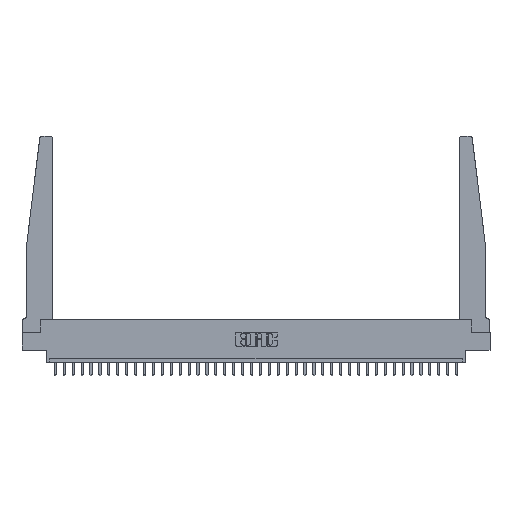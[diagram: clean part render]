
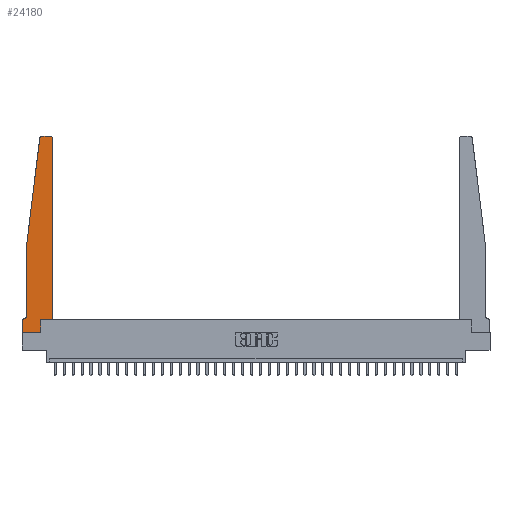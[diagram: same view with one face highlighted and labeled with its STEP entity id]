
A CAD part, top view. The second image highlights one B-rep face of the part: STEP entity #24180.
In plain terms, the highlighted planar face has unit normal (0, 0, 1).
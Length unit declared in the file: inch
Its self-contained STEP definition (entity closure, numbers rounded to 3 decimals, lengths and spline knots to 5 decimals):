
#249 = VERTEX_POINT ( 'NONE', #25269 ) ;
#447 = ORIENTED_EDGE ( 'NONE', *, *, #11841, .T. ) ;
#845 = CARTESIAN_POINT ( 'NONE',  ( 0.2605, 0.18, 0.37 ) ) ;
#974 = CARTESIAN_POINT ( 'NONE',  ( 0.27653, 2.75, 0.37 ) ) ;
#1027 = ORIENTED_EDGE ( 'NONE', *, *, #14362, .T. ) ;
#1041 = ORIENTED_EDGE ( 'NONE', *, *, #11023, .T. ) ;
#1573 = LINE ( 'NONE', #22048, #18857 ) ;
#1698 = CARTESIAN_POINT ( 'NONE',  ( 0.015, 0.1875, 0.37 ) ) ;
#2093 = ORIENTED_EDGE ( 'NONE', *, *, #29009, .T. ) ;
#2115 = VERTEX_POINT ( 'NONE', #1698 ) ;
#2901 = EDGE_CURVE ( 'NONE', #2115, #19477, #16508, .T. ) ;
#3150 = EDGE_CURVE ( 'NONE', #9063, #27293, #18668, .T. ) ;
#3406 = VECTOR ( 'NONE', #26445, 39.37008 ) ;
#3407 = ORIENTED_EDGE ( 'NONE', *, *, #17997, .T. ) ;
#3594 = LINE ( 'NONE', #24094, #30791 ) ;
#4368 = CARTESIAN_POINT ( 'NONE',  ( 0., 0., 0.37 ) ) ;
#4501 = DIRECTION ( 'NONE',  ( 1., 0., 0. ) ) ;
#6658 = LINE ( 'NONE', #21712, #22932 ) ;
#7038 = CARTESIAN_POINT ( 'NONE',  ( 0., 0.1875, 0.37 ) ) ;
#7677 = CARTESIAN_POINT ( 'NONE',  ( 0.2605, 0., 0.37 ) ) ;
#7689 = DIRECTION ( 'NONE',  ( 1., 0., 0. ) ) ;
#8015 = DIRECTION ( 'NONE',  ( 0., 0., 1. ) ) ;
#8926 = DIRECTION ( 'NONE',  ( -1., 0., 0. ) ) ;
#9063 = VERTEX_POINT ( 'NONE', #10203 ) ;
#9131 = AXIS2_PLACEMENT_3D ( 'NONE', #18800, #19141, #29138 ) ;
#9810 = VECTOR ( 'NONE', #16277, 39.37008 ) ;
#10203 = CARTESIAN_POINT ( 'NONE',  ( 0.425, 2.72, 0.37 ) ) ;
#10653 = LINE ( 'NONE', #18788, #18963 ) ;
#11023 = EDGE_CURVE ( 'NONE', #27715, #249, #14028, .T. ) ;
#11247 = CARTESIAN_POINT ( 'NONE',  ( 0.425, 0.18, 0.37 ) ) ;
#11837 = CARTESIAN_POINT ( 'NONE',  ( 0.425, 0.18, 0.37 ) ) ;
#11841 = EDGE_CURVE ( 'NONE', #27293, #32899, #18833, .T. ) ;
#12548 = AXIS2_PLACEMENT_3D ( 'NONE', #32112, #26361, #8926 ) ;
#14028 = LINE ( 'NONE', #11837, #29240 ) ;
#14362 = EDGE_CURVE ( 'NONE', #21719, #2115, #32006, .T. ) ;
#14790 = EDGE_CURVE ( 'NONE', #249, #9063, #18699, .T. ) ;
#14977 = PLANE ( 'NONE',  #32138 ) ;
#15306 = EDGE_CURVE ( 'NONE', #23309, #19709, #28999, .T. ) ;
#16064 = DIRECTION ( 'NONE',  ( 1., 0., 0. ) ) ;
#16275 = CARTESIAN_POINT ( 'NONE',  ( 0.395, 2.75, 0.37 ) ) ;
#16277 = DIRECTION ( 'NONE',  ( -1., 0., 0. ) ) ;
#16382 = VERTEX_POINT ( 'NONE', #7677 ) ;
#16490 = DIRECTION ( 'NONE',  ( 0., 1., 0. ) ) ;
#16508 = LINE ( 'NONE', #27013, #17019 ) ;
#16528 = EDGE_CURVE ( 'NONE', #19477, #22649, #3594, .T. ) ;
#17019 = VECTOR ( 'NONE', #32258, 39.37008 ) ;
#17597 = ORIENTED_EDGE ( 'NONE', *, *, #2901, .T. ) ;
#17843 = ORIENTED_EDGE ( 'NONE', *, *, #16528, .T. ) ;
#17997 = EDGE_CURVE ( 'NONE', #22649, #16382, #10653, .T. ) ;
#18668 = CIRCLE ( 'NONE', #26778, 0.03 ) ;
#18699 = LINE ( 'NONE', #11247, #27184 ) ;
#18788 = CARTESIAN_POINT ( 'NONE',  ( 0., 0., 0.37 ) ) ;
#18800 = CARTESIAN_POINT ( 'NONE',  ( 0.27653, 2.72, 0.37 ) ) ;
#18833 = LINE ( 'NONE', #21528, #9810 ) ;
#18857 = VECTOR ( 'NONE', #19178, 39.37008 ) ;
#18963 = VECTOR ( 'NONE', #16064, 39.37008 ) ;
#19141 = DIRECTION ( 'NONE',  ( 0., 0., 1. ) ) ;
#19178 = DIRECTION ( 'NONE',  ( 0., 1., 0. ) ) ;
#19477 = VERTEX_POINT ( 'NONE', #27939 ) ;
#19709 = VERTEX_POINT ( 'NONE', #28593 ) ;
#19768 = EDGE_LOOP ( 'NONE', ( #447, #24705, #22943, #21004, #1027, #17597, #17843, #3407, #2093, #1041, #32133, #27331 ) ) ;
#21004 = ORIENTED_EDGE ( 'NONE', *, *, #21642, .T. ) ;
#21528 = CARTESIAN_POINT ( 'NONE',  ( 0.25, 2.75, 0.37 ) ) ;
#21642 = EDGE_CURVE ( 'NONE', #19709, #21719, #6658, .T. ) ;
#21712 = CARTESIAN_POINT ( 'NONE',  ( 0.065, 1.25, 0.37 ) ) ;
#21719 = VERTEX_POINT ( 'NONE', #24272 ) ;
#22048 = CARTESIAN_POINT ( 'NONE',  ( 0.2605, 0.18, 0.37 ) ) ;
#22649 = VERTEX_POINT ( 'NONE', #4368 ) ;
#22777 = DIRECTION ( 'NONE',  ( 0., 0., 1. ) ) ;
#22932 = VECTOR ( 'NONE', #26808, 39.37008 ) ;
#22943 = ORIENTED_EDGE ( 'NONE', *, *, #15306, .T. ) ;
#23309 = VERTEX_POINT ( 'NONE', #30153 ) ;
#23715 = CIRCLE ( 'NONE', #9131, 0.03 ) ;
#24094 = CARTESIAN_POINT ( 'NONE',  ( 0., 0., 0.37 ) ) ;
#24180 = ADVANCED_FACE ( 'NONE', ( #27874 ), #14977, .T. ) ;
#24272 = CARTESIAN_POINT ( 'NONE',  ( 0.065, 0.2375, 0.37 ) ) ;
#24705 = ORIENTED_EDGE ( 'NONE', *, *, #29475, .T. ) ;
#25269 = CARTESIAN_POINT ( 'NONE',  ( 0.425, 0.18, 0.37 ) ) ;
#26361 = DIRECTION ( 'NONE',  ( 0., 0., -1. ) ) ;
#26445 = DIRECTION ( 'NONE',  ( -0.122, -0.992, 0. ) ) ;
#26615 = CARTESIAN_POINT ( 'NONE',  ( 0.065, 1.25, 0.37 ) ) ;
#26778 = AXIS2_PLACEMENT_3D ( 'NONE', #28679, #8015, #7689 ) ;
#26797 = DIRECTION ( 'NONE',  ( 0., -1., 0. ) ) ;
#26808 = DIRECTION ( 'NONE',  ( 0., -1., 0. ) ) ;
#27013 = CARTESIAN_POINT ( 'NONE',  ( 0.065, 0.1875, 0.37 ) ) ;
#27184 = VECTOR ( 'NONE', #16490, 39.37008 ) ;
#27293 = VERTEX_POINT ( 'NONE', #16275 ) ;
#27331 = ORIENTED_EDGE ( 'NONE', *, *, #3150, .T. ) ;
#27715 = VERTEX_POINT ( 'NONE', #845 ) ;
#27874 = FACE_OUTER_BOUND ( 'NONE', #19768, .T. ) ;
#27939 = CARTESIAN_POINT ( 'NONE',  ( 0., 0.1875, 0.37 ) ) ;
#28593 = CARTESIAN_POINT ( 'NONE',  ( 0.065, 1.25, 0.37 ) ) ;
#28679 = CARTESIAN_POINT ( 'NONE',  ( 0.395, 2.72, 0.37 ) ) ;
#28999 = LINE ( 'NONE', #26615, #3406 ) ;
#29009 = EDGE_CURVE ( 'NONE', #16382, #27715, #1573, .T. ) ;
#29138 = DIRECTION ( 'NONE',  ( 1., 0., 0. ) ) ;
#29240 = VECTOR ( 'NONE', #30127, 39.37008 ) ;
#29475 = EDGE_CURVE ( 'NONE', #32899, #23309, #23715, .T. ) ;
#30127 = DIRECTION ( 'NONE',  ( 1., 0., 0. ) ) ;
#30153 = CARTESIAN_POINT ( 'NONE',  ( 0.24675, 2.72367, 0.37 ) ) ;
#30791 = VECTOR ( 'NONE', #26797, 39.37008 ) ;
#32006 = CIRCLE ( 'NONE', #12548, 0.05 ) ;
#32112 = CARTESIAN_POINT ( 'NONE',  ( 0.015, 0.2375, 0.37 ) ) ;
#32133 = ORIENTED_EDGE ( 'NONE', *, *, #14790, .T. ) ;
#32138 = AXIS2_PLACEMENT_3D ( 'NONE', #7038, #22777, #4501 ) ;
#32258 = DIRECTION ( 'NONE',  ( -1., 0., 0. ) ) ;
#32899 = VERTEX_POINT ( 'NONE', #974 ) ;
